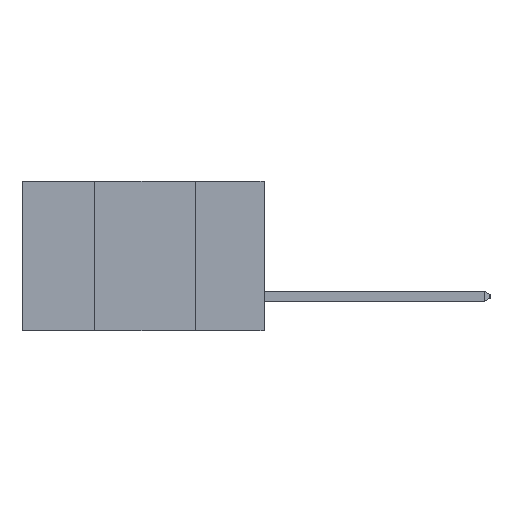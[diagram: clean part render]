
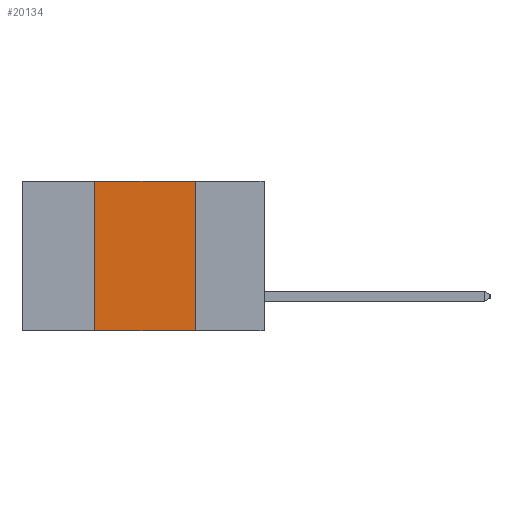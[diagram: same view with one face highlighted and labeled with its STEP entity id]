
A CAD part, left-side view. The second image highlights one B-rep face of the part: STEP entity #20134.
In plain terms, the highlighted planar face has unit normal (-1, 0, 0).
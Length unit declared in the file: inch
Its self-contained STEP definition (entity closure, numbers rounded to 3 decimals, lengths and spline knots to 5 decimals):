
#16 = VECTOR ( 'NONE', #16762, 39.37008 ) ;
#87 = EDGE_CURVE ( 'NONE', #4935, #23399, #20089, .T. ) ;
#140 = CARTESIAN_POINT ( 'NONE',  ( 0., 0.6, 0. ) ) ;
#512 = ORIENTED_EDGE ( 'NONE', *, *, #87, .T. ) ;
#786 = VECTOR ( 'NONE', #24487, 39.37008 ) ;
#1867 = ORIENTED_EDGE ( 'NONE', *, *, #13735, .F. ) ;
#1889 = FACE_OUTER_BOUND ( 'NONE', #2329, .T. ) ;
#1966 = VERTEX_POINT ( 'NONE', #6870 ) ;
#2054 = CARTESIAN_POINT ( 'NONE',  ( 0., 0.17, -0.37 ) ) ;
#2329 = EDGE_LOOP ( 'NONE', ( #1867, #16810, #8915, #512 ) ) ;
#3744 = VECTOR ( 'NONE', #13742, 39.37008 ) ;
#4240 = DIRECTION ( 'NONE',  ( 1., 0., 0. ) ) ;
#4935 = VERTEX_POINT ( 'NONE', #20058 ) ;
#6870 = CARTESIAN_POINT ( 'NONE',  ( 0., 0.42, 0. ) ) ;
#7471 = CARTESIAN_POINT ( 'NONE',  ( 0., 0.42, -0.37 ) ) ;
#8915 = ORIENTED_EDGE ( 'NONE', *, *, #18865, .F. ) ;
#9809 = VERTEX_POINT ( 'NONE', #21425 ) ;
#9855 = DIRECTION ( 'NONE',  ( 0., -1., 0. ) ) ;
#10041 = PLANE ( 'NONE',  #15703 ) ;
#10162 = CARTESIAN_POINT ( 'NONE',  ( 0., 0.6, -0.37 ) ) ;
#13735 = EDGE_CURVE ( 'NONE', #9809, #23399, #14059, .T. ) ;
#13742 = DIRECTION ( 'NONE',  ( 0., 0., -1. ) ) ;
#14059 = LINE ( 'NONE', #2054, #3744 ) ;
#15010 = EDGE_CURVE ( 'NONE', #1966, #9809, #16833, .T. ) ;
#15703 = AXIS2_PLACEMENT_3D ( 'NONE', #140, #4240, #17705 ) ;
#16220 = VECTOR ( 'NONE', #9855, 39.37008 ) ;
#16358 = LINE ( 'NONE', #7471, #786 ) ;
#16762 = DIRECTION ( 'NONE',  ( 0., -1., 0. ) ) ;
#16810 = ORIENTED_EDGE ( 'NONE', *, *, #15010, .F. ) ;
#16833 = LINE ( 'NONE', #24876, #16220 ) ;
#17705 = DIRECTION ( 'NONE',  ( 0., 0., -1. ) ) ;
#18865 = EDGE_CURVE ( 'NONE', #4935, #1966, #16358, .T. ) ;
#20058 = CARTESIAN_POINT ( 'NONE',  ( 0., 0.42, -0.37 ) ) ;
#20089 = LINE ( 'NONE', #10162, #16 ) ;
#20134 = ADVANCED_FACE ( 'NONE', ( #1889 ), #10041, .F. ) ;
#21425 = CARTESIAN_POINT ( 'NONE',  ( 0., 0.17, 0. ) ) ;
#21631 = CARTESIAN_POINT ( 'NONE',  ( 0., 0.17, -0.37 ) ) ;
#23399 = VERTEX_POINT ( 'NONE', #21631 ) ;
#24487 = DIRECTION ( 'NONE',  ( 0., 0., 1. ) ) ;
#24876 = CARTESIAN_POINT ( 'NONE',  ( 0., 0.6, 0. ) ) ;
